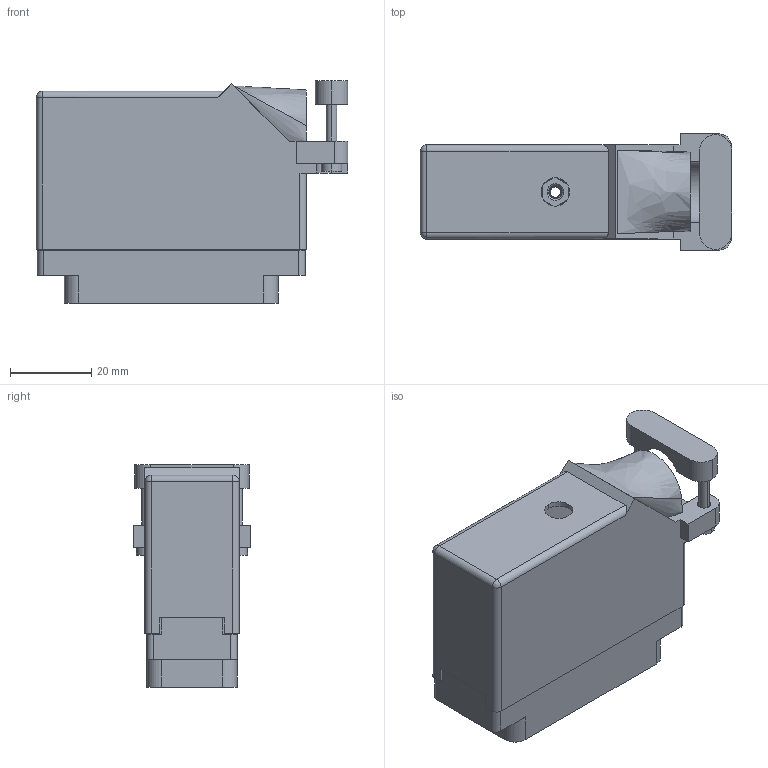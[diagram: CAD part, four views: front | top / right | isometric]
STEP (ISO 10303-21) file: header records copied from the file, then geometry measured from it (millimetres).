
FILE_DESCRIPTION (( 'STEP AP203' ), '1' );
FILE_NAME ('516-056-000-346.STEP', '2020-03-10T04:44:29', ( '' ), ( '' ), 'SwSTEP 2.0', 'SolidWorks 2016', '' );
FILE_SCHEMA (( 'CONFIG_CONTROL_DESIGN' ));
Length unit declared in the file: inch
Products named in the file (4): 516-230-001_Plastic - 056 Side Entry - Large Clamp; 516-056-000-346; 516 Plug Insulator_056; 516-252-035-100_516-252-035-100
Assembly tree (3 placements, depth 2):
  516-056-000-346
    516 Plug Insulator_056
    516-230-001_Plastic - 056 Side Entry - Large Clamp
    516-252-035-100_516-252-035-100
Bounding box: 76.5 x 28.57 x 54.69 mm (x, y, z)
Volume: 24260.5 mm3; surface area: 32991.8 mm2
Topology: 3 solids, 3 shells, 1352 faces, 3952 edges, 2628 vertices
Faces by surface type: plane 953, cylinder 376, cone 12, bspline 9, sphere 2
Entity records: 47803 total; most frequent: CARTESIAN_POINT 10475, ORIENTED_EDGE 7900, DIRECTION 7557, EDGE_CURVE 3950, LINE 2933, VECTOR 2933, VERTEX_POINT 2628, AXIS2_PLACEMENT_3D 2312
